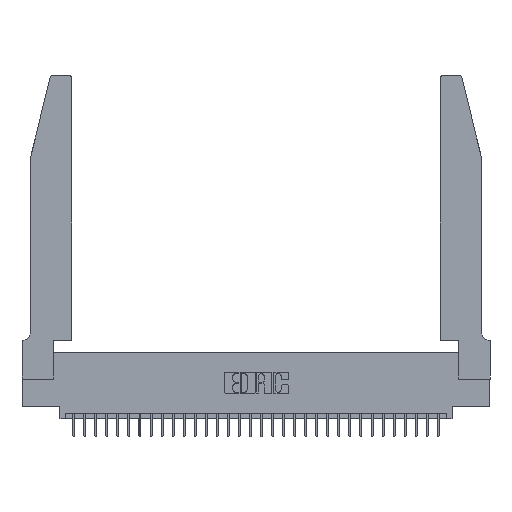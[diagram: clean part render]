
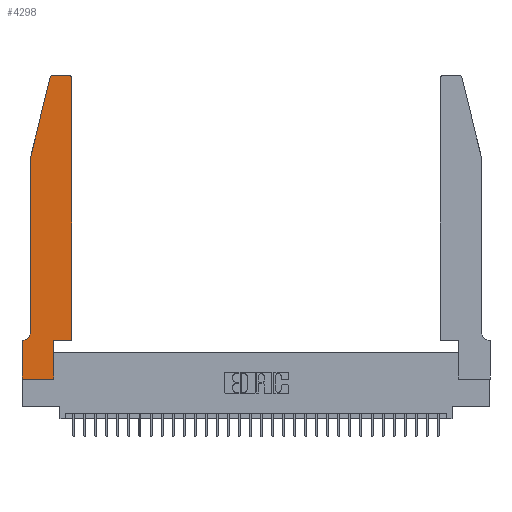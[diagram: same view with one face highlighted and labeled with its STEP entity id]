
A CAD part, top view. The second image highlights one B-rep face of the part: STEP entity #4298.
In plain terms, the highlighted planar face has unit normal (0, 0, 1).
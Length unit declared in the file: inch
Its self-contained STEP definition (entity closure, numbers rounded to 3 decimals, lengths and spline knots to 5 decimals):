
#94 = ORIENTED_EDGE ( 'NONE', *, *, #12276, .T. ) ;
#943 = CARTESIAN_POINT ( 'NONE',  ( 0., 0.35, 0.37 ) ) ;
#1545 = CARTESIAN_POINT ( 'NONE',  ( 0.0755, 2., 0.37 ) ) ;
#1922 = CIRCLE ( 'NONE', #17203, 0.03 ) ;
#2031 = EDGE_CURVE ( 'NONE', #4310, #5520, #2413, .T. ) ;
#2413 = LINE ( 'NONE', #30713, #2775 ) ;
#2415 = CARTESIAN_POINT ( 'NONE',  ( 0.4505, 0.35, 0.37 ) ) ;
#2556 = DIRECTION ( 'NONE',  ( 0., 0., 1. ) ) ;
#2645 = ORIENTED_EDGE ( 'NONE', *, *, #28124, .T. ) ;
#2664 = DIRECTION ( 'NONE',  ( 1., 0., 0. ) ) ;
#2775 = VECTOR ( 'NONE', #31160, 39.37008 ) ;
#2789 = VERTEX_POINT ( 'NONE', #15260 ) ;
#3289 = ORIENTED_EDGE ( 'NONE', *, *, #15527, .T. ) ;
#3521 = LINE ( 'NONE', #10517, #20513 ) ;
#3779 = CARTESIAN_POINT ( 'NONE',  ( 0.25487, 2.72718, 0.37 ) ) ;
#4298 = ADVANCED_FACE ( 'NONE', ( #4608 ), #15150, .T. ) ;
#4310 = VERTEX_POINT ( 'NONE', #22803 ) ;
#4608 = FACE_OUTER_BOUND ( 'NONE', #25841, .T. ) ;
#5510 = LINE ( 'NONE', #17889, #10654 ) ;
#5520 = VERTEX_POINT ( 'NONE', #19040 ) ;
#5872 = CIRCLE ( 'NONE', #13717, 0.03 ) ;
#6048 = AXIS2_PLACEMENT_3D ( 'NONE', #17796, #2556, #2664 ) ;
#6322 = VECTOR ( 'NONE', #22362, 39.37008 ) ;
#7549 = DIRECTION ( 'NONE',  ( 1., 0., 0. ) ) ;
#8343 = CARTESIAN_POINT ( 'NONE',  ( 0.0755, 2., 0.37 ) ) ;
#8539 = VERTEX_POINT ( 'NONE', #10691 ) ;
#8812 = VERTEX_POINT ( 'NONE', #943 ) ;
#9444 = ORIENTED_EDGE ( 'NONE', *, *, #16463, .T. ) ;
#9659 = CARTESIAN_POINT ( 'NONE',  ( 0.2865, 0.35, 0.37 ) ) ;
#10010 = DIRECTION ( 'NONE',  ( 0., 0., -1. ) ) ;
#10517 = CARTESIAN_POINT ( 'NONE',  ( 0.0755, 0.35, 0.37 ) ) ;
#10654 = VECTOR ( 'NONE', #7549, 39.37008 ) ;
#10691 = CARTESIAN_POINT ( 'NONE',  ( 0.2865, 0., 0.37 ) ) ;
#11230 = EDGE_CURVE ( 'NONE', #2789, #8539, #5510, .T. ) ;
#11384 = ORIENTED_EDGE ( 'NONE', *, *, #17548, .T. ) ;
#11412 = DIRECTION ( 'NONE',  ( -1., 0., 0. ) ) ;
#11415 = VERTEX_POINT ( 'NONE', #24917 ) ;
#11451 = ORIENTED_EDGE ( 'NONE', *, *, #15455, .T. ) ;
#11993 = CARTESIAN_POINT ( 'NONE',  ( 0., 0., 0.37 ) ) ;
#12108 = EDGE_CURVE ( 'NONE', #5520, #11415, #5872, .T. ) ;
#12276 = EDGE_CURVE ( 'NONE', #11415, #31600, #13337, .T. ) ;
#12432 = DIRECTION ( 'NONE',  ( 0., -1., 0. ) ) ;
#12560 = DIRECTION ( 'NONE',  ( 1., 0., 0. ) ) ;
#13195 = VERTEX_POINT ( 'NONE', #9659 ) ;
#13296 = VERTEX_POINT ( 'NONE', #3779 ) ;
#13337 = LINE ( 'NONE', #21615, #31151 ) ;
#13717 = AXIS2_PLACEMENT_3D ( 'NONE', #31320, #26352, #18838 ) ;
#14271 = VECTOR ( 'NONE', #31824, 39.37008 ) ;
#14635 = EDGE_CURVE ( 'NONE', #13296, #23576, #21025, .T. ) ;
#15040 = EDGE_CURVE ( 'NONE', #8539, #13195, #24548, .T. ) ;
#15150 = PLANE ( 'NONE',  #6048 ) ;
#15260 = CARTESIAN_POINT ( 'NONE',  ( 0., 0., 0.37 ) ) ;
#15270 = VECTOR ( 'NONE', #12560, 39.37008 ) ;
#15421 = ORIENTED_EDGE ( 'NONE', *, *, #12108, .T. ) ;
#15455 = EDGE_CURVE ( 'NONE', #8812, #2789, #16590, .T. ) ;
#15527 = EDGE_CURVE ( 'NONE', #24482, #8812, #3521, .T. ) ;
#16266 = CARTESIAN_POINT ( 'NONE',  ( 0.0755, 0.42, 0.37 ) ) ;
#16463 = EDGE_CURVE ( 'NONE', #23576, #31370, #18519, .T. ) ;
#16590 = LINE ( 'NONE', #11993, #20951 ) ;
#17203 = AXIS2_PLACEMENT_3D ( 'NONE', #31501, #21371, #23791 ) ;
#17548 = EDGE_CURVE ( 'NONE', #13195, #4310, #27954, .T. ) ;
#17796 = CARTESIAN_POINT ( 'NONE',  ( 0., 0.35, 0.37 ) ) ;
#17889 = CARTESIAN_POINT ( 'NONE',  ( 0., 0., 0.37 ) ) ;
#18226 = DIRECTION ( 'NONE',  ( -1., 0., 0. ) ) ;
#18519 = LINE ( 'NONE', #22525, #19345 ) ;
#18838 = DIRECTION ( 'NONE',  ( 1., 0., 0. ) ) ;
#19040 = CARTESIAN_POINT ( 'NONE',  ( 0.4505, 2.72, 0.37 ) ) ;
#19345 = VECTOR ( 'NONE', #12432, 39.37008 ) ;
#19913 = CARTESIAN_POINT ( 'NONE',  ( 0.284, 2.75, 0.37 ) ) ;
#20513 = VECTOR ( 'NONE', #18226, 39.37008 ) ;
#20951 = VECTOR ( 'NONE', #29690, 39.37008 ) ;
#21025 = LINE ( 'NONE', #1545, #14271 ) ;
#21371 = DIRECTION ( 'NONE',  ( 0., 0., 1. ) ) ;
#21615 = CARTESIAN_POINT ( 'NONE',  ( 0.2605, 2.75, 0.37 ) ) ;
#22362 = DIRECTION ( 'NONE',  ( 0., 1., 0. ) ) ;
#22525 = CARTESIAN_POINT ( 'NONE',  ( 0.0755, 2., 0.37 ) ) ;
#22558 = ORIENTED_EDGE ( 'NONE', *, *, #2031, .T. ) ;
#22803 = CARTESIAN_POINT ( 'NONE',  ( 0.4505, 0.35, 0.37 ) ) ;
#22851 = CARTESIAN_POINT ( 'NONE',  ( 0.0055, 0.42, 0.37 ) ) ;
#23576 = VERTEX_POINT ( 'NONE', #8343 ) ;
#23791 = DIRECTION ( 'NONE',  ( 1., 0., 0. ) ) ;
#24482 = VERTEX_POINT ( 'NONE', #31512 ) ;
#24548 = LINE ( 'NONE', #32376, #6322 ) ;
#24677 = CIRCLE ( 'NONE', #28229, 0.07 ) ;
#24917 = CARTESIAN_POINT ( 'NONE',  ( 0.4205, 2.75, 0.37 ) ) ;
#25841 = EDGE_LOOP ( 'NONE', ( #94, #26845, #29810, #9444, #2645, #3289, #11451, #27573, #32521, #11384, #22558, #15421 ) ) ;
#26352 = DIRECTION ( 'NONE',  ( 0., 0., 1. ) ) ;
#26636 = EDGE_CURVE ( 'NONE', #31600, #13296, #1922, .T. ) ;
#26845 = ORIENTED_EDGE ( 'NONE', *, *, #26636, .T. ) ;
#27573 = ORIENTED_EDGE ( 'NONE', *, *, #11230, .T. ) ;
#27715 = DIRECTION ( 'NONE',  ( -1., 0., 0. ) ) ;
#27954 = LINE ( 'NONE', #2415, #15270 ) ;
#28124 = EDGE_CURVE ( 'NONE', #31370, #24482, #24677, .T. ) ;
#28229 = AXIS2_PLACEMENT_3D ( 'NONE', #22851, #10010, #27715 ) ;
#29690 = DIRECTION ( 'NONE',  ( 0., -1., 0. ) ) ;
#29810 = ORIENTED_EDGE ( 'NONE', *, *, #14635, .T. ) ;
#30713 = CARTESIAN_POINT ( 'NONE',  ( 0.4505, 0.35, 0.37 ) ) ;
#31151 = VECTOR ( 'NONE', #11412, 39.37008 ) ;
#31160 = DIRECTION ( 'NONE',  ( 0., 1., 0. ) ) ;
#31320 = CARTESIAN_POINT ( 'NONE',  ( 0.4205, 2.72, 0.37 ) ) ;
#31370 = VERTEX_POINT ( 'NONE', #16266 ) ;
#31501 = CARTESIAN_POINT ( 'NONE',  ( 0.284, 2.72, 0.37 ) ) ;
#31512 = CARTESIAN_POINT ( 'NONE',  ( 0.0055, 0.35, 0.37 ) ) ;
#31600 = VERTEX_POINT ( 'NONE', #19913 ) ;
#31824 = DIRECTION ( 'NONE',  ( -0.239, -0.971, 0. ) ) ;
#32376 = CARTESIAN_POINT ( 'NONE',  ( 0.2865, 0.35, 0.37 ) ) ;
#32521 = ORIENTED_EDGE ( 'NONE', *, *, #15040, .T. ) ;
